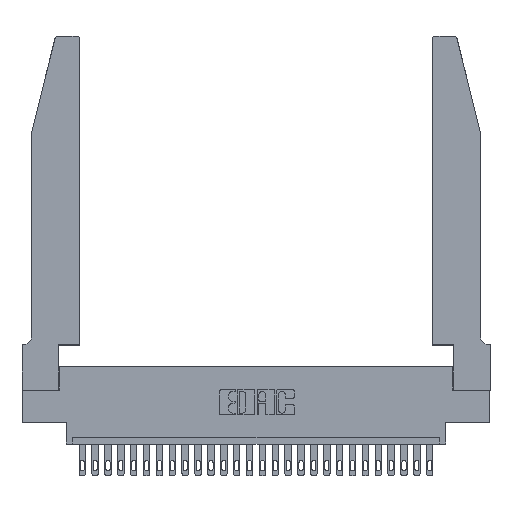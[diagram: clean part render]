
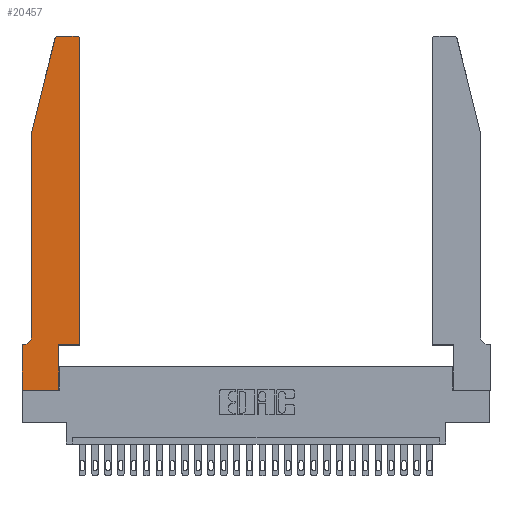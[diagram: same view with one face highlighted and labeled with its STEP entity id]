
A CAD part, top view. The second image highlights one B-rep face of the part: STEP entity #20457.
In plain terms, the highlighted planar face has unit normal (0, 0, 1).
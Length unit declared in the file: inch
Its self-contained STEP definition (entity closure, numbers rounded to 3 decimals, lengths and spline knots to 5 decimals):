
#9 = CARTESIAN_POINT ( 'NONE',  ( 0.4505, 2.72, 0.37 ) ) ;
#24 = DIRECTION ( 'NONE',  ( 1., 0., 0. ) ) ;
#58 = CIRCLE ( 'NONE', #17083, 0.03 ) ;
#270 = ORIENTED_EDGE ( 'NONE', *, *, #12567, .T. ) ;
#1035 = LINE ( 'NONE', #22465, #25842 ) ;
#1038 = CARTESIAN_POINT ( 'NONE',  ( 0.0755, 0.42, 0.37 ) ) ;
#1123 = ORIENTED_EDGE ( 'NONE', *, *, #8641, .T. ) ;
#1442 = EDGE_CURVE ( 'NONE', #4483, #8779, #13116, .T. ) ;
#1629 = CARTESIAN_POINT ( 'NONE',  ( 0., 0., 0.37 ) ) ;
#2195 = ORIENTED_EDGE ( 'NONE', *, *, #25710, .T. ) ;
#2740 = CARTESIAN_POINT ( 'NONE',  ( 0.0055, 0.35, 0.37 ) ) ;
#2884 = AXIS2_PLACEMENT_3D ( 'NONE', #25879, #21450, #12889 ) ;
#2951 = DIRECTION ( 'NONE',  ( 0., 1., 0. ) ) ;
#3472 = ORIENTED_EDGE ( 'NONE', *, *, #1442, .T. ) ;
#3701 = EDGE_CURVE ( 'NONE', #15341, #15634, #11663, .T. ) ;
#4087 = DIRECTION ( 'NONE',  ( 0., -1., 0. ) ) ;
#4137 = DIRECTION ( 'NONE',  ( 0., -1., 0. ) ) ;
#4191 = CARTESIAN_POINT ( 'NONE',  ( 0.0755, 0.35, 0.37 ) ) ;
#4241 = VERTEX_POINT ( 'NONE', #23608 ) ;
#4267 = VERTEX_POINT ( 'NONE', #17237 ) ;
#4483 = VERTEX_POINT ( 'NONE', #18333 ) ;
#4519 = EDGE_CURVE ( 'NONE', #16361, #4483, #21000, .T. ) ;
#4940 = DIRECTION ( 'NONE',  ( -0.239, -0.971, 0. ) ) ;
#5099 = VERTEX_POINT ( 'NONE', #9 ) ;
#5157 = CARTESIAN_POINT ( 'NONE',  ( 0., 0.35, 0.37 ) ) ;
#5452 = VECTOR ( 'NONE', #9998, 39.37008 ) ;
#5488 = VERTEX_POINT ( 'NONE', #26553 ) ;
#5516 = FACE_OUTER_BOUND ( 'NONE', #19917, .T. ) ;
#5654 = CARTESIAN_POINT ( 'NONE',  ( 0.2865, 0.35, 0.37 ) ) ;
#6182 = VERTEX_POINT ( 'NONE', #12335 ) ;
#7443 = EDGE_CURVE ( 'NONE', #5488, #15583, #18505, .T. ) ;
#7576 = LINE ( 'NONE', #8562, #17555 ) ;
#7694 = EDGE_CURVE ( 'NONE', #6182, #18588, #11124, .T. ) ;
#8372 = CIRCLE ( 'NONE', #25399, 0.07 ) ;
#8480 = DIRECTION ( 'NONE',  ( 1., 0., 0. ) ) ;
#8518 = CARTESIAN_POINT ( 'NONE',  ( 0.4205, 2.72, 0.37 ) ) ;
#8562 = CARTESIAN_POINT ( 'NONE',  ( 0.0755, 2., 0.37 ) ) ;
#8641 = EDGE_CURVE ( 'NONE', #4241, #5099, #1035, .T. ) ;
#8779 = VERTEX_POINT ( 'NONE', #21652 ) ;
#9785 = LINE ( 'NONE', #25524, #22807 ) ;
#9910 = ORIENTED_EDGE ( 'NONE', *, *, #4519, .T. ) ;
#9998 = DIRECTION ( 'NONE',  ( 0., 1., 0. ) ) ;
#10133 = CARTESIAN_POINT ( 'NONE',  ( 0.0755, 2., 0.37 ) ) ;
#10668 = DIRECTION ( 'NONE',  ( 1., 0., 0. ) ) ;
#10838 = ORIENTED_EDGE ( 'NONE', *, *, #21751, .T. ) ;
#11001 = VECTOR ( 'NONE', #13416, 39.37008 ) ;
#11124 = LINE ( 'NONE', #20434, #5452 ) ;
#11663 = LINE ( 'NONE', #4191, #11001 ) ;
#12335 = CARTESIAN_POINT ( 'NONE',  ( 0.2865, 0., 0.37 ) ) ;
#12567 = EDGE_CURVE ( 'NONE', #8779, #5488, #7576, .T. ) ;
#12708 = CARTESIAN_POINT ( 'NONE',  ( 0.0055, 0.42, 0.37 ) ) ;
#12857 = VECTOR ( 'NONE', #4137, 39.37008 ) ;
#12889 = DIRECTION ( 'NONE',  ( 1., 0., 0. ) ) ;
#13116 = CIRCLE ( 'NONE', #21981, 0.03 ) ;
#13416 = DIRECTION ( 'NONE',  ( -1., 0., 0. ) ) ;
#15341 = VERTEX_POINT ( 'NONE', #2740 ) ;
#15583 = VERTEX_POINT ( 'NONE', #1038 ) ;
#15634 = VERTEX_POINT ( 'NONE', #5157 ) ;
#15654 = EDGE_CURVE ( 'NONE', #4267, #6182, #22429, .T. ) ;
#16317 = ORIENTED_EDGE ( 'NONE', *, *, #7443, .T. ) ;
#16361 = VERTEX_POINT ( 'NONE', #25106 ) ;
#16444 = ORIENTED_EDGE ( 'NONE', *, *, #19962, .T. ) ;
#16479 = ORIENTED_EDGE ( 'NONE', *, *, #23797, .T. ) ;
#17083 = AXIS2_PLACEMENT_3D ( 'NONE', #8518, #23448, #10668 ) ;
#17237 = CARTESIAN_POINT ( 'NONE',  ( 0., 0., 0.37 ) ) ;
#17522 = ORIENTED_EDGE ( 'NONE', *, *, #15654, .T. ) ;
#17555 = VECTOR ( 'NONE', #4940, 39.37008 ) ;
#18333 = CARTESIAN_POINT ( 'NONE',  ( 0.284, 2.75, 0.37 ) ) ;
#18505 = LINE ( 'NONE', #10133, #12857 ) ;
#18588 = VERTEX_POINT ( 'NONE', #5654 ) ;
#18820 = DIRECTION ( 'NONE',  ( 0., 0., 1. ) ) ;
#19096 = VECTOR ( 'NONE', #24786, 39.37008 ) ;
#19917 = EDGE_LOOP ( 'NONE', ( #9910, #3472, #270, #16317, #2195, #26877, #16444, #17522, #21109, #10838, #1123, #16479 ) ) ;
#19962 = EDGE_CURVE ( 'NONE', #15634, #4267, #21266, .T. ) ;
#20296 = VECTOR ( 'NONE', #24839, 39.37008 ) ;
#20434 = CARTESIAN_POINT ( 'NONE',  ( 0.2865, 0.35, 0.37 ) ) ;
#20457 = ADVANCED_FACE ( 'NONE', ( #5516 ), #21543, .T. ) ;
#21000 = LINE ( 'NONE', #22208, #20296 ) ;
#21109 = ORIENTED_EDGE ( 'NONE', *, *, #7694, .T. ) ;
#21256 = CARTESIAN_POINT ( 'NONE',  ( 0.284, 2.72, 0.37 ) ) ;
#21266 = LINE ( 'NONE', #27493, #25322 ) ;
#21450 = DIRECTION ( 'NONE',  ( 0., 0., 1. ) ) ;
#21543 = PLANE ( 'NONE',  #2884 ) ;
#21652 = CARTESIAN_POINT ( 'NONE',  ( 0.25487, 2.72718, 0.37 ) ) ;
#21751 = EDGE_CURVE ( 'NONE', #18588, #4241, #9785, .T. ) ;
#21981 = AXIS2_PLACEMENT_3D ( 'NONE', #21256, #18820, #8480 ) ;
#22208 = CARTESIAN_POINT ( 'NONE',  ( 0.2605, 2.75, 0.37 ) ) ;
#22429 = LINE ( 'NONE', #1629, #19096 ) ;
#22465 = CARTESIAN_POINT ( 'NONE',  ( 0.4505, 0.35, 0.37 ) ) ;
#22807 = VECTOR ( 'NONE', #24, 39.37008 ) ;
#23448 = DIRECTION ( 'NONE',  ( 0., 0., 1. ) ) ;
#23608 = CARTESIAN_POINT ( 'NONE',  ( 0.4505, 0.35, 0.37 ) ) ;
#23797 = EDGE_CURVE ( 'NONE', #5099, #16361, #58, .T. ) ;
#24786 = DIRECTION ( 'NONE',  ( 1., 0., 0. ) ) ;
#24839 = DIRECTION ( 'NONE',  ( -1., 0., 0. ) ) ;
#25106 = CARTESIAN_POINT ( 'NONE',  ( 0.4205, 2.75, 0.37 ) ) ;
#25322 = VECTOR ( 'NONE', #4087, 39.37008 ) ;
#25399 = AXIS2_PLACEMENT_3D ( 'NONE', #12708, #27688, #25619 ) ;
#25524 = CARTESIAN_POINT ( 'NONE',  ( 0.4505, 0.35, 0.37 ) ) ;
#25619 = DIRECTION ( 'NONE',  ( -1., 0., 0. ) ) ;
#25710 = EDGE_CURVE ( 'NONE', #15583, #15341, #8372, .T. ) ;
#25842 = VECTOR ( 'NONE', #2951, 39.37008 ) ;
#25879 = CARTESIAN_POINT ( 'NONE',  ( 0., 0.35, 0.37 ) ) ;
#26553 = CARTESIAN_POINT ( 'NONE',  ( 0.0755, 2., 0.37 ) ) ;
#26877 = ORIENTED_EDGE ( 'NONE', *, *, #3701, .T. ) ;
#27493 = CARTESIAN_POINT ( 'NONE',  ( 0., 0., 0.37 ) ) ;
#27688 = DIRECTION ( 'NONE',  ( 0., 0., -1. ) ) ;
